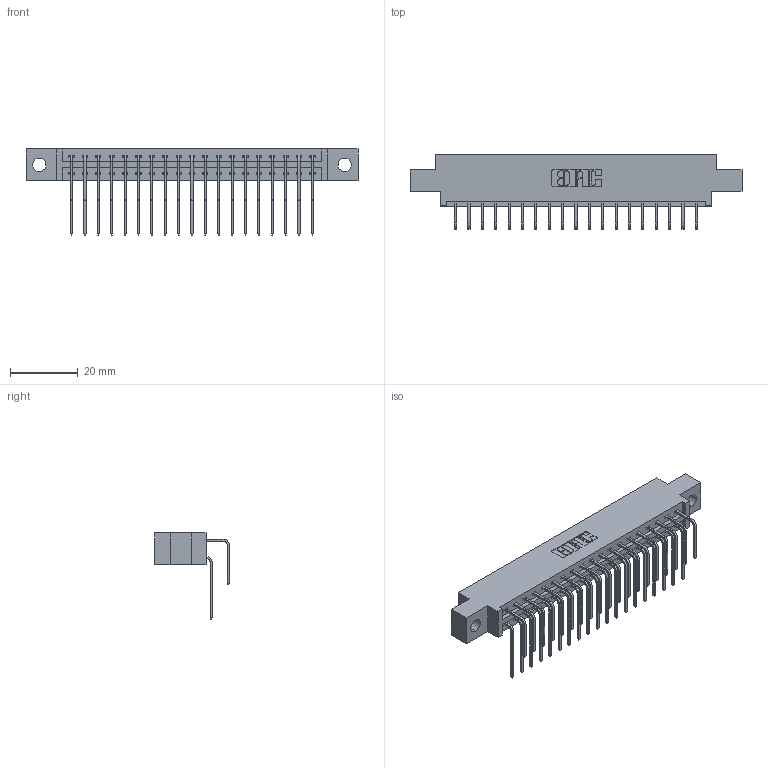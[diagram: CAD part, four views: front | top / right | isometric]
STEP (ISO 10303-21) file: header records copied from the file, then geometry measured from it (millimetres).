
FILE_DESCRIPTION (( 'STEP AP203' ), '1' );
FILE_NAME ('337-038-558-804.STEP', '2018-08-08T05:51:46', ( '' ), ( '' ), 'SwSTEP 2.0', 'SolidWorks 2016', '' );
FILE_SCHEMA (( 'CONFIG_CONTROL_DESIGN' ));
Length unit declared in the file: inch
Products named in the file (4): 337 Part_0.170 Offset - 0.156 Dia-TH; 345-292-001_558 559 Tail - 1; 345-292-001_558 Tail - 2; 337-038-558-804
Assembly tree (39 placements, depth 2):
  337-038-558-804
    337 Part_0.170 Offset - 0.156 Dia-TH
    345-292-001_558 559 Tail - 1  x19
    345-292-001_558 Tail - 2  x19
Bounding box: 98.3 x 22.17 x 25.53 mm (x, y, z)
Volume: 10067.1 mm3; surface area: 12163.4 mm2
Topology: 39 solids, 39 shells, 2246 faces, 6669 edges, 4394 vertices
Faces by surface type: plane 1594, cylinder 652
Entity records: 19625 total; most frequent: CARTESIAN_POINT 3373, ORIENTED_EDGE 3258, DIRECTION 2893, EDGE_CURVE 1629, VECTOR 1461, LINE 1461, VERTEX_POINT 1082, AXIS2_PLACEMENT_3D 716
